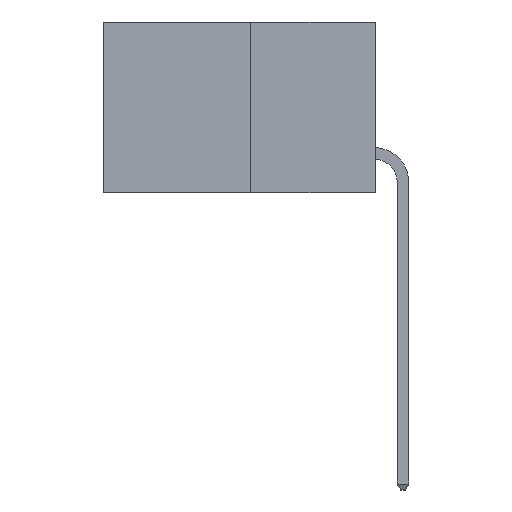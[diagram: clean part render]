
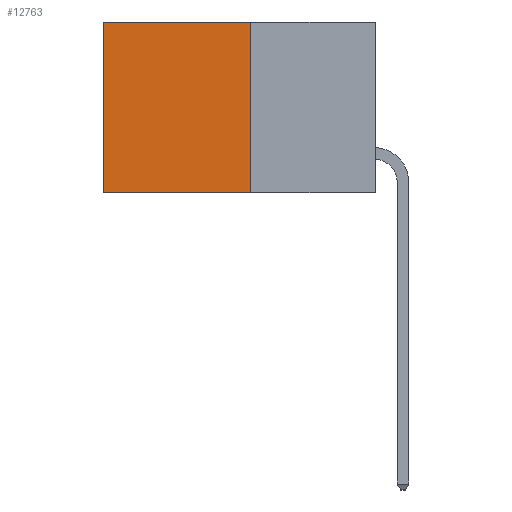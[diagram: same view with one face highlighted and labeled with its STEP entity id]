
A CAD part, left-side view. The second image highlights one B-rep face of the part: STEP entity #12763.
In plain terms, the highlighted planar face has unit normal (-1, 0, 0).
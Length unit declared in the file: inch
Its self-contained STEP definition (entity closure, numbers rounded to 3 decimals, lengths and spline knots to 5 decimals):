
#2 = DIRECTION ( 'NONE',  ( 1., 0., 0. ) ) ;
#1594 = LINE ( 'NONE', #5254, #10797 ) ;
#1840 = LINE ( 'NONE', #21990, #15589 ) ;
#2186 = EDGE_CURVE ( 'NONE', #3030, #3408, #21721, .T. ) ;
#2694 = CARTESIAN_POINT ( 'NONE',  ( 0.277, 0.59, -0.37 ) ) ;
#3030 = VERTEX_POINT ( 'NONE', #20629 ) ;
#3408 = VERTEX_POINT ( 'NONE', #11387 ) ;
#3999 = ORIENTED_EDGE ( 'NONE', *, *, #8897, .F. ) ;
#4535 = EDGE_CURVE ( 'NONE', #3408, #19626, #16825, .T. ) ;
#5254 = CARTESIAN_POINT ( 'NONE',  ( 0.277, 0.27, -0.37 ) ) ;
#5676 = ORIENTED_EDGE ( 'NONE', *, *, #4535, .T. ) ;
#5731 = DIRECTION ( 'NONE',  ( 0., 0., -1. ) ) ;
#6029 = CARTESIAN_POINT ( 'NONE',  ( 0.277, 0.59, -0.37 ) ) ;
#6402 = AXIS2_PLACEMENT_3D ( 'NONE', #11115, #2, #12850 ) ;
#8639 = VECTOR ( 'NONE', #18188, 39.37008 ) ;
#8897 = EDGE_CURVE ( 'NONE', #14317, #19626, #1840, .T. ) ;
#9325 = EDGE_LOOP ( 'NONE', ( #5676, #3999, #19080, #21699 ) ) ;
#10797 = VECTOR ( 'NONE', #15818, 39.37008 ) ;
#11115 = CARTESIAN_POINT ( 'NONE',  ( 0.277, 0.27, -0.37 ) ) ;
#11387 = CARTESIAN_POINT ( 'NONE',  ( 0.277, 0.59, 0. ) ) ;
#12763 = ADVANCED_FACE ( 'NONE', ( #14171 ), #16212, .F. ) ;
#12850 = DIRECTION ( 'NONE',  ( 0., 0., -1. ) ) ;
#14171 = FACE_OUTER_BOUND ( 'NONE', #9325, .T. ) ;
#14317 = VERTEX_POINT ( 'NONE', #20031 ) ;
#15264 = EDGE_CURVE ( 'NONE', #3030, #14317, #1594, .T. ) ;
#15589 = VECTOR ( 'NONE', #20321, 39.37008 ) ;
#15818 = DIRECTION ( 'NONE',  ( 0., 0., -1. ) ) ;
#16212 = PLANE ( 'NONE',  #6402 ) ;
#16308 = VECTOR ( 'NONE', #5731, 39.37008 ) ;
#16825 = LINE ( 'NONE', #6029, #16308 ) ;
#18188 = DIRECTION ( 'NONE',  ( 0., 1., 0. ) ) ;
#19080 = ORIENTED_EDGE ( 'NONE', *, *, #15264, .F. ) ;
#19626 = VERTEX_POINT ( 'NONE', #2694 ) ;
#19713 = CARTESIAN_POINT ( 'NONE',  ( 0.277, 0.27, 0. ) ) ;
#20031 = CARTESIAN_POINT ( 'NONE',  ( 0.277, 0.27, -0.37 ) ) ;
#20321 = DIRECTION ( 'NONE',  ( 0., 1., 0. ) ) ;
#20629 = CARTESIAN_POINT ( 'NONE',  ( 0.277, 0.27, 0. ) ) ;
#21699 = ORIENTED_EDGE ( 'NONE', *, *, #2186, .T. ) ;
#21721 = LINE ( 'NONE', #19713, #8639 ) ;
#21990 = CARTESIAN_POINT ( 'NONE',  ( 0.277, 0.27, -0.37 ) ) ;
